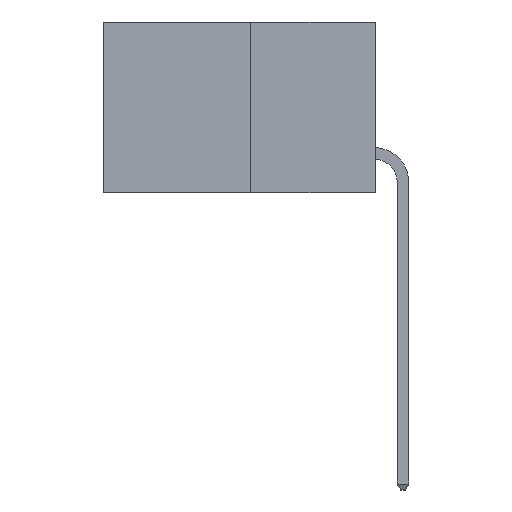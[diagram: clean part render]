
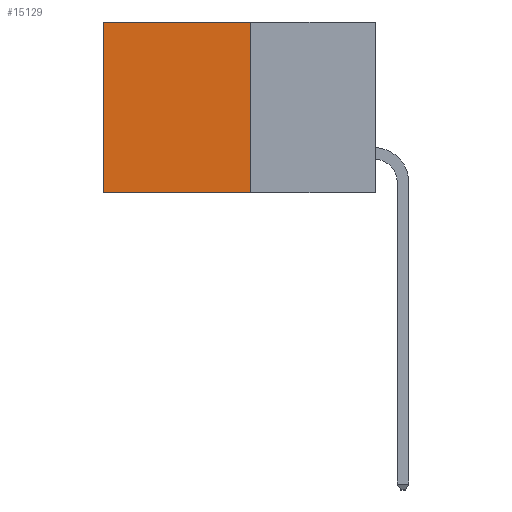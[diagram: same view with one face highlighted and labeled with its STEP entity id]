
A CAD part, left-side view. The second image highlights one B-rep face of the part: STEP entity #15129.
In plain terms, the highlighted planar face has unit normal (-1, 0, 0).
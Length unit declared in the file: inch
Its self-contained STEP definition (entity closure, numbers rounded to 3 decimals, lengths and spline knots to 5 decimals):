
#659 = DIRECTION ( 'NONE',  ( 0., 0., -1. ) ) ;
#1199 = ORIENTED_EDGE ( 'NONE', *, *, #13975, .F. ) ;
#1224 = LINE ( 'NONE', #18902, #4720 ) ;
#3273 = VECTOR ( 'NONE', #16303, 39.37008 ) ;
#3475 = LINE ( 'NONE', #14869, #3273 ) ;
#4164 = VERTEX_POINT ( 'NONE', #14086 ) ;
#4532 = CARTESIAN_POINT ( 'NONE',  ( 0.277, 0.27, 0. ) ) ;
#4720 = VECTOR ( 'NONE', #16054, 39.37008 ) ;
#5010 = EDGE_LOOP ( 'NONE', ( #14368, #1199, #17440, #12186 ) ) ;
#5083 = CARTESIAN_POINT ( 'NONE',  ( 0.277, 0.27, -0.37 ) ) ;
#5278 = CARTESIAN_POINT ( 'NONE',  ( 0.277, 0.59, -0.37 ) ) ;
#5330 = AXIS2_PLACEMENT_3D ( 'NONE', #5083, #9490, #659 ) ;
#6350 = CARTESIAN_POINT ( 'NONE',  ( 0.277, 0.27, -0.37 ) ) ;
#7826 = DIRECTION ( 'NONE',  ( 0., 0., -1. ) ) ;
#8849 = VECTOR ( 'NONE', #7826, 39.37008 ) ;
#9490 = DIRECTION ( 'NONE',  ( 1., 0., 0. ) ) ;
#9541 = EDGE_CURVE ( 'NONE', #4164, #9937, #12266, .T. ) ;
#9770 = CARTESIAN_POINT ( 'NONE',  ( 0.277, 0.59, 0. ) ) ;
#9937 = VERTEX_POINT ( 'NONE', #13070 ) ;
#12186 = ORIENTED_EDGE ( 'NONE', *, *, #17664, .T. ) ;
#12266 = LINE ( 'NONE', #6350, #8849 ) ;
#12496 = VERTEX_POINT ( 'NONE', #9770 ) ;
#13070 = CARTESIAN_POINT ( 'NONE',  ( 0.277, 0.27, -0.37 ) ) ;
#13687 = VERTEX_POINT ( 'NONE', #5278 ) ;
#13975 = EDGE_CURVE ( 'NONE', #9937, #13687, #1224, .T. ) ;
#14086 = CARTESIAN_POINT ( 'NONE',  ( 0.277, 0.27, 0. ) ) ;
#14368 = ORIENTED_EDGE ( 'NONE', *, *, #15550, .T. ) ;
#14405 = LINE ( 'NONE', #4532, #17785 ) ;
#14869 = CARTESIAN_POINT ( 'NONE',  ( 0.277, 0.59, -0.37 ) ) ;
#15129 = ADVANCED_FACE ( 'NONE', ( #15169 ), #18153, .F. ) ;
#15169 = FACE_OUTER_BOUND ( 'NONE', #5010, .T. ) ;
#15550 = EDGE_CURVE ( 'NONE', #12496, #13687, #3475, .T. ) ;
#16054 = DIRECTION ( 'NONE',  ( 0., 1., 0. ) ) ;
#16163 = DIRECTION ( 'NONE',  ( 0., 1., 0. ) ) ;
#16303 = DIRECTION ( 'NONE',  ( 0., 0., -1. ) ) ;
#17440 = ORIENTED_EDGE ( 'NONE', *, *, #9541, .F. ) ;
#17664 = EDGE_CURVE ( 'NONE', #4164, #12496, #14405, .T. ) ;
#17785 = VECTOR ( 'NONE', #16163, 39.37008 ) ;
#18153 = PLANE ( 'NONE',  #5330 ) ;
#18902 = CARTESIAN_POINT ( 'NONE',  ( 0.277, 0.27, -0.37 ) ) ;
